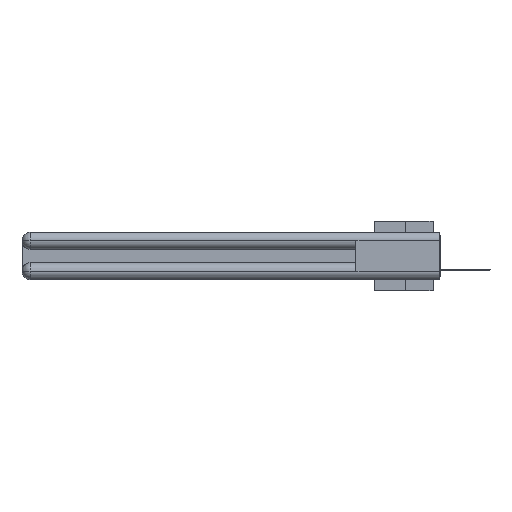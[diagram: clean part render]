
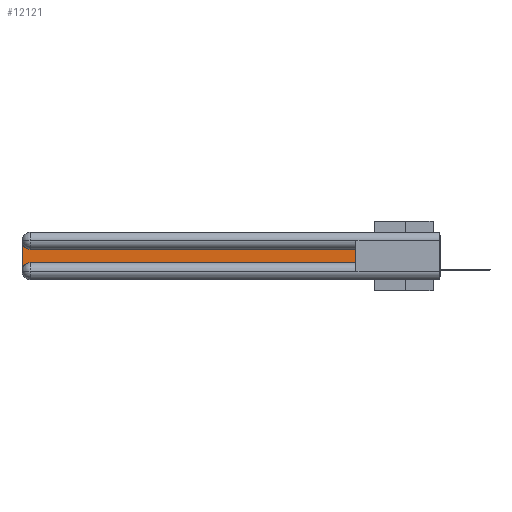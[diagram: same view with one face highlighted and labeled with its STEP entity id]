
A CAD part, left-side view. The second image highlights one B-rep face of the part: STEP entity #12121.
In plain terms, the highlighted planar face has unit normal (-1, 0, 0).
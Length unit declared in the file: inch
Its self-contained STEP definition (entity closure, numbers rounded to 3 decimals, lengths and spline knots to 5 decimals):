
#1291 = CARTESIAN_POINT ( 'NONE',  ( 0.075, 0.6, -0.2175 ) ) ;
#1433 = AXIS2_PLACEMENT_3D ( 'NONE', #17030, #26206, #36935 ) ;
#5178 = CARTESIAN_POINT ( 'NONE',  ( 0.075, 3., -0.0625 ) ) ;
#5439 = EDGE_CURVE ( 'NONE', #33105, #27881, #17674, .T. ) ;
#6565 = LINE ( 'NONE', #1291, #22358 ) ;
#8448 = CARTESIAN_POINT ( 'NONE',  ( 0.075, 0.6, -0.2175 ) ) ;
#9696 = DIRECTION ( 'NONE',  ( 1., 0., 0. ) ) ;
#9741 = LINE ( 'NONE', #27025, #18829 ) ;
#10240 = VERTEX_POINT ( 'NONE', #21183 ) ;
#10436 = CARTESIAN_POINT ( 'NONE',  ( 0.075, 2.94, -0.2775 ) ) ;
#10585 = FACE_OUTER_BOUND ( 'NONE', #20998, .T. ) ;
#11563 = VERTEX_POINT ( 'NONE', #18008 ) ;
#11695 = CIRCLE ( 'NONE', #12889, 0.06 ) ;
#11749 = LINE ( 'NONE', #29037, #21813 ) ;
#12121 = ADVANCED_FACE ( 'NONE', ( #10585 ), #28064, .F. ) ;
#12494 = ORIENTED_EDGE ( 'NONE', *, *, #18080, .T. ) ;
#12889 = AXIS2_PLACEMENT_3D ( 'NONE', #10436, #9696, #21550 ) ;
#14887 = ORIENTED_EDGE ( 'NONE', *, *, #20458, .T. ) ;
#15016 = EDGE_CURVE ( 'NONE', #10240, #33105, #11749, .T. ) ;
#15876 = CARTESIAN_POINT ( 'NONE',  ( 0.075, 3., -0.1225 ) ) ;
#16045 = EDGE_CURVE ( 'NONE', #19618, #10240, #6565, .T. ) ;
#17030 = CARTESIAN_POINT ( 'NONE',  ( 0.075, 2.94, -0.0625 ) ) ;
#17674 = CIRCLE ( 'NONE', #1433, 0.06 ) ;
#18008 = CARTESIAN_POINT ( 'NONE',  ( 0.075, 2.94, -0.2175 ) ) ;
#18080 = EDGE_CURVE ( 'NONE', #18097, #11563, #11695, .T. ) ;
#18097 = VERTEX_POINT ( 'NONE', #27360 ) ;
#18626 = AXIS2_PLACEMENT_3D ( 'NONE', #15876, #27326, #19072 ) ;
#18805 = CARTESIAN_POINT ( 'NONE',  ( 0.075, 2.94, -0.1225 ) ) ;
#18829 = VECTOR ( 'NONE', #23839, 39.37008 ) ;
#19072 = DIRECTION ( 'NONE',  ( 0., 0., -1. ) ) ;
#19531 = ORIENTED_EDGE ( 'NONE', *, *, #5439, .T. ) ;
#19618 = VERTEX_POINT ( 'NONE', #20411 ) ;
#20411 = CARTESIAN_POINT ( 'NONE',  ( 0.075, 0.6, -0.2175 ) ) ;
#20458 = EDGE_CURVE ( 'NONE', #11563, #19618, #22207, .T. ) ;
#20998 = EDGE_LOOP ( 'NONE', ( #35885, #19531, #27972, #12494, #14887, #35366 ) ) ;
#21183 = CARTESIAN_POINT ( 'NONE',  ( 0.075, 0.6, -0.1225 ) ) ;
#21343 = EDGE_CURVE ( 'NONE', #27881, #18097, #9741, .T. ) ;
#21550 = DIRECTION ( 'NONE',  ( 0., 0., -1. ) ) ;
#21766 = VECTOR ( 'NONE', #33660, 39.37008 ) ;
#21813 = VECTOR ( 'NONE', #26390, 39.37008 ) ;
#22207 = LINE ( 'NONE', #8448, #21766 ) ;
#22358 = VECTOR ( 'NONE', #26679, 39.37008 ) ;
#23839 = DIRECTION ( 'NONE',  ( 0., 0., -1. ) ) ;
#26206 = DIRECTION ( 'NONE',  ( 1., 0., 0. ) ) ;
#26390 = DIRECTION ( 'NONE',  ( 0., 1., 0. ) ) ;
#26679 = DIRECTION ( 'NONE',  ( 0., 0., 1. ) ) ;
#27025 = CARTESIAN_POINT ( 'NONE',  ( 0.075, 3., -0.2175 ) ) ;
#27326 = DIRECTION ( 'NONE',  ( 1., 0., 0. ) ) ;
#27360 = CARTESIAN_POINT ( 'NONE',  ( 0.075, 3., -0.2775 ) ) ;
#27881 = VERTEX_POINT ( 'NONE', #5178 ) ;
#27972 = ORIENTED_EDGE ( 'NONE', *, *, #21343, .T. ) ;
#28064 = PLANE ( 'NONE',  #18626 ) ;
#29037 = CARTESIAN_POINT ( 'NONE',  ( 0.075, 0.6, -0.1225 ) ) ;
#33105 = VERTEX_POINT ( 'NONE', #18805 ) ;
#33660 = DIRECTION ( 'NONE',  ( 0., -1., 0. ) ) ;
#35366 = ORIENTED_EDGE ( 'NONE', *, *, #16045, .T. ) ;
#35885 = ORIENTED_EDGE ( 'NONE', *, *, #15016, .T. ) ;
#36935 = DIRECTION ( 'NONE',  ( 0., 0., -1. ) ) ;
